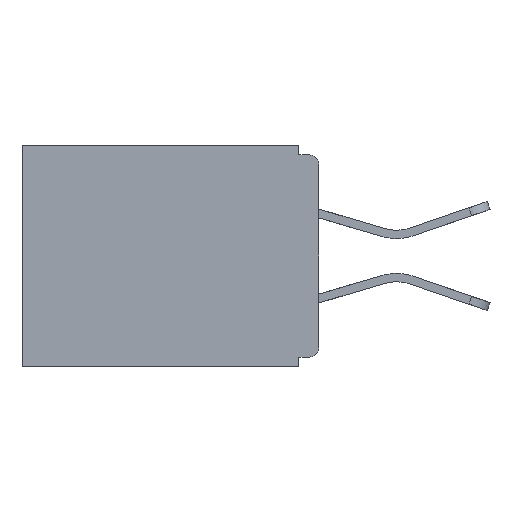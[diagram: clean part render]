
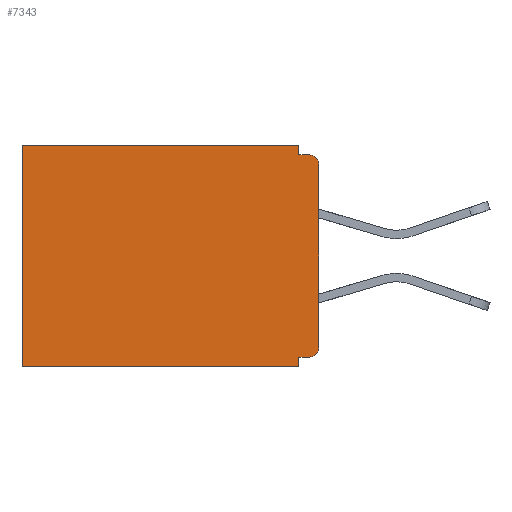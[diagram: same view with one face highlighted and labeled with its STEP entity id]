
A CAD part, left-side view. The second image highlights one B-rep face of the part: STEP entity #7343.
In plain terms, the highlighted planar face has unit normal (-1, 0, 0).
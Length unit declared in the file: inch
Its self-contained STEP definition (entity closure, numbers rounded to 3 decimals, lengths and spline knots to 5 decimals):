
#151 = VECTOR ( 'NONE', #8135, 39.37008 ) ;
#255 = DIRECTION ( 'NONE',  ( 1., 0., 0. ) ) ;
#512 = VERTEX_POINT ( 'NONE', #7494 ) ;
#602 = VERTEX_POINT ( 'NONE', #10117 ) ;
#949 = LINE ( 'NONE', #6033, #5334 ) ;
#1197 = DIRECTION ( 'NONE',  ( 0., 1., 0. ) ) ;
#1253 = EDGE_LOOP ( 'NONE', ( #11065, #2351, #10294, #11894, #5116, #11267, #5986, #2775, #1828, #10566 ) ) ;
#1743 = FACE_OUTER_BOUND ( 'NONE', #1253, .T. ) ;
#1781 = CARTESIAN_POINT ( 'NONE',  ( 0.298, 0., -0.313 ) ) ;
#1828 = ORIENTED_EDGE ( 'NONE', *, *, #8807, .T. ) ;
#1983 = VERTEX_POINT ( 'NONE', #1781 ) ;
#2062 = DIRECTION ( 'NONE',  ( 0., 0., -1. ) ) ;
#2351 = ORIENTED_EDGE ( 'NONE', *, *, #11836, .F. ) ;
#2562 = EDGE_CURVE ( 'NONE', #7207, #1983, #6797, .T. ) ;
#2584 = EDGE_CURVE ( 'NONE', #2983, #11001, #6645, .T. ) ;
#2651 = DIRECTION ( 'NONE',  ( 0., -1., 0. ) ) ;
#2686 = CARTESIAN_POINT ( 'NONE',  ( 0.298, 0.031, -0.343 ) ) ;
#2775 = ORIENTED_EDGE ( 'NONE', *, *, #8848, .F. ) ;
#2839 = VERTEX_POINT ( 'NONE', #9420 ) ;
#2916 = EDGE_CURVE ( 'NONE', #11001, #9690, #6315, .T. ) ;
#2983 = VERTEX_POINT ( 'NONE', #12047 ) ;
#3071 = LINE ( 'NONE', #9717, #7653 ) ;
#3088 = CARTESIAN_POINT ( 'NONE',  ( 0.298, 0.015, -0.313 ) ) ;
#3106 = CARTESIAN_POINT ( 'NONE',  ( 0.298, 0., 0. ) ) ;
#3144 = DIRECTION ( 'NONE',  ( 0., 0., -1. ) ) ;
#3564 = CARTESIAN_POINT ( 'NONE',  ( 0.298, 0., -0.03 ) ) ;
#3941 = DIRECTION ( 'NONE',  ( 0., 0., -1. ) ) ;
#3959 = VECTOR ( 'NONE', #9299, 39.37008 ) ;
#4040 = PLANE ( 'NONE',  #7507 ) ;
#4074 = DIRECTION ( 'NONE',  ( 0., 1., 0. ) ) ;
#4095 = VECTOR ( 'NONE', #10330, 39.37008 ) ;
#4287 = LINE ( 'NONE', #8140, #7875 ) ;
#4332 = VECTOR ( 'NONE', #1197, 39.37008 ) ;
#4641 = VERTEX_POINT ( 'NONE', #9181 ) ;
#4989 = LINE ( 'NONE', #2686, #3959 ) ;
#4993 = VERTEX_POINT ( 'NONE', #10240 ) ;
#5116 = ORIENTED_EDGE ( 'NONE', *, *, #2916, .T. ) ;
#5334 = VECTOR ( 'NONE', #8107, 39.37008 ) ;
#5437 = EDGE_CURVE ( 'NONE', #2983, #2839, #949, .T. ) ;
#5986 = ORIENTED_EDGE ( 'NONE', *, *, #7187, .F. ) ;
#5991 = CARTESIAN_POINT ( 'NONE',  ( 0.298, 0.015, -0.03 ) ) ;
#6014 = CARTESIAN_POINT ( 'NONE',  ( 0.298, 0., 0. ) ) ;
#6033 = CARTESIAN_POINT ( 'NONE',  ( 0.298, 0.031, -0.343 ) ) ;
#6315 = LINE ( 'NONE', #8099, #151 ) ;
#6415 = EDGE_CURVE ( 'NONE', #7207, #512, #12100, .T. ) ;
#6645 = LINE ( 'NONE', #8483, #4095 ) ;
#6797 = LINE ( 'NONE', #6014, #7071 ) ;
#6855 = CARTESIAN_POINT ( 'NONE',  ( 0.298, 0., -0.328 ) ) ;
#6911 = CIRCLE ( 'NONE', #11314, 0.015 ) ;
#6922 = CARTESIAN_POINT ( 'NONE',  ( 0.298, 0.46, -0.343 ) ) ;
#6946 = DIRECTION ( 'NONE',  ( -1., 0., 0. ) ) ;
#7071 = VECTOR ( 'NONE', #2062, 39.37008 ) ;
#7187 = EDGE_CURVE ( 'NONE', #4641, #4993, #4989, .T. ) ;
#7207 = VERTEX_POINT ( 'NONE', #3564 ) ;
#7343 = ADVANCED_FACE ( 'NONE', ( #1743 ), #4040, .F. ) ;
#7494 = CARTESIAN_POINT ( 'NONE',  ( 0.298, 0.015, -0.015 ) ) ;
#7507 = AXIS2_PLACEMENT_3D ( 'NONE', #3106, #255, #3144 ) ;
#7653 = VECTOR ( 'NONE', #4074, 39.37008 ) ;
#7756 = DIRECTION ( 'NONE',  ( -1., 0., 0. ) ) ;
#7875 = VECTOR ( 'NONE', #2651, 39.37008 ) ;
#8099 = CARTESIAN_POINT ( 'NONE',  ( 0.298, 0.46, 0. ) ) ;
#8107 = DIRECTION ( 'NONE',  ( 0., 0., -1. ) ) ;
#8135 = DIRECTION ( 'NONE',  ( 0., 0., -1. ) ) ;
#8140 = CARTESIAN_POINT ( 'NONE',  ( 0.298, 0., -0.015 ) ) ;
#8228 = EDGE_CURVE ( 'NONE', #4993, #9690, #3071, .T. ) ;
#8384 = AXIS2_PLACEMENT_3D ( 'NONE', #5991, #6946, #11579 ) ;
#8483 = CARTESIAN_POINT ( 'NONE',  ( 0.298, 0., 0. ) ) ;
#8585 = CARTESIAN_POINT ( 'NONE',  ( 0.298, 0.46, 0. ) ) ;
#8807 = EDGE_CURVE ( 'NONE', #602, #1983, #6911, .T. ) ;
#8848 = EDGE_CURVE ( 'NONE', #602, #4641, #11738, .T. ) ;
#9181 = CARTESIAN_POINT ( 'NONE',  ( 0.298, 0.031, -0.328 ) ) ;
#9299 = DIRECTION ( 'NONE',  ( 0., 0., -1. ) ) ;
#9420 = CARTESIAN_POINT ( 'NONE',  ( 0.298, 0.031, -0.015 ) ) ;
#9690 = VERTEX_POINT ( 'NONE', #6922 ) ;
#9717 = CARTESIAN_POINT ( 'NONE',  ( 0.298, 0., -0.343 ) ) ;
#10117 = CARTESIAN_POINT ( 'NONE',  ( 0.298, 0.015, -0.328 ) ) ;
#10240 = CARTESIAN_POINT ( 'NONE',  ( 0.298, 0.031, -0.343 ) ) ;
#10294 = ORIENTED_EDGE ( 'NONE', *, *, #5437, .F. ) ;
#10330 = DIRECTION ( 'NONE',  ( 0., 1., 0. ) ) ;
#10566 = ORIENTED_EDGE ( 'NONE', *, *, #2562, .F. ) ;
#11001 = VERTEX_POINT ( 'NONE', #8585 ) ;
#11065 = ORIENTED_EDGE ( 'NONE', *, *, #6415, .T. ) ;
#11267 = ORIENTED_EDGE ( 'NONE', *, *, #8228, .F. ) ;
#11314 = AXIS2_PLACEMENT_3D ( 'NONE', #3088, #7756, #3941 ) ;
#11579 = DIRECTION ( 'NONE',  ( 0., 0., -1. ) ) ;
#11738 = LINE ( 'NONE', #6855, #4332 ) ;
#11836 = EDGE_CURVE ( 'NONE', #2839, #512, #4287, .T. ) ;
#11894 = ORIENTED_EDGE ( 'NONE', *, *, #2584, .T. ) ;
#12047 = CARTESIAN_POINT ( 'NONE',  ( 0.298, 0.031, 0. ) ) ;
#12100 = CIRCLE ( 'NONE', #8384, 0.015 ) ;
